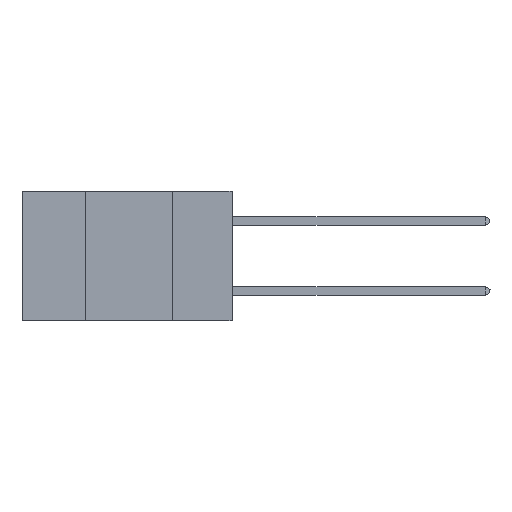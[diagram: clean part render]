
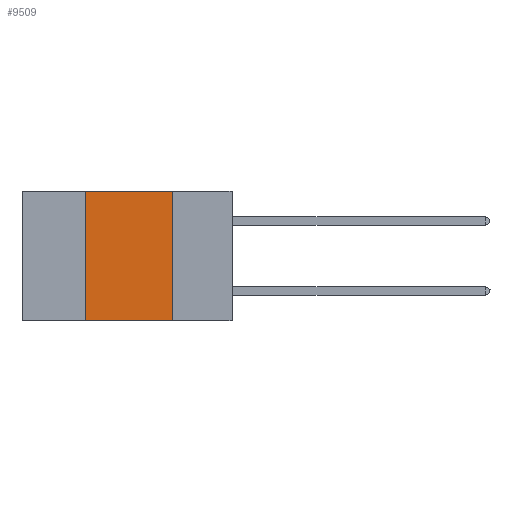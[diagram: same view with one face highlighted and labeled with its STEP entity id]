
A CAD part, left-side view. The second image highlights one B-rep face of the part: STEP entity #9509.
In plain terms, the highlighted planar face has unit normal (-1, 0, 0).
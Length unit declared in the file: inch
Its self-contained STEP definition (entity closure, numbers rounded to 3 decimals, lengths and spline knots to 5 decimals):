
#65 = DIRECTION ( 'NONE',  ( 0., -1., 0. ) ) ;
#109 = DIRECTION ( 'NONE',  ( 0., 0., -1. ) ) ;
#229 = VERTEX_POINT ( 'NONE', #6644 ) ;
#1941 = CARTESIAN_POINT ( 'NONE',  ( 0., 0.42, 0. ) ) ;
#2054 = VERTEX_POINT ( 'NONE', #14027 ) ;
#2383 = DIRECTION ( 'NONE',  ( 0., 0., 1. ) ) ;
#2789 = CARTESIAN_POINT ( 'NONE',  ( 0., 0.6, -0.37 ) ) ;
#3727 = VECTOR ( 'NONE', #12505, 39.37008 ) ;
#3840 = AXIS2_PLACEMENT_3D ( 'NONE', #13118, #4748, #14555 ) ;
#4183 = CARTESIAN_POINT ( 'NONE',  ( 0., 0.17, -0.37 ) ) ;
#4316 = LINE ( 'NONE', #12627, #7850 ) ;
#4524 = LINE ( 'NONE', #2789, #14394 ) ;
#4748 = DIRECTION ( 'NONE',  ( 1., 0., 0. ) ) ;
#4802 = ORIENTED_EDGE ( 'NONE', *, *, #10144, .T. ) ;
#6644 = CARTESIAN_POINT ( 'NONE',  ( 0., 0.42, -0.37 ) ) ;
#7850 = VECTOR ( 'NONE', #109, 39.37008 ) ;
#8315 = FACE_OUTER_BOUND ( 'NONE', #8778, .T. ) ;
#8761 = VERTEX_POINT ( 'NONE', #9739 ) ;
#8778 = EDGE_LOOP ( 'NONE', ( #17605, #14218, #14602, #4802 ) ) ;
#9509 = ADVANCED_FACE ( 'NONE', ( #8315 ), #10340, .F. ) ;
#9739 = CARTESIAN_POINT ( 'NONE',  ( 0., 0.42, 0. ) ) ;
#10140 = EDGE_CURVE ( 'NONE', #2054, #14435, #4316, .T. ) ;
#10144 = EDGE_CURVE ( 'NONE', #229, #14435, #4524, .T. ) ;
#10340 = PLANE ( 'NONE',  #3840 ) ;
#10991 = CARTESIAN_POINT ( 'NONE',  ( 0., 0.6, 0. ) ) ;
#12238 = LINE ( 'NONE', #1941, #13791 ) ;
#12505 = DIRECTION ( 'NONE',  ( 0., -1., 0. ) ) ;
#12627 = CARTESIAN_POINT ( 'NONE',  ( 0., 0.17, 0. ) ) ;
#13118 = CARTESIAN_POINT ( 'NONE',  ( 0., 0.6, 0. ) ) ;
#13791 = VECTOR ( 'NONE', #2383, 39.37008 ) ;
#14027 = CARTESIAN_POINT ( 'NONE',  ( 0., 0.17, 0. ) ) ;
#14218 = ORIENTED_EDGE ( 'NONE', *, *, #15514, .F. ) ;
#14394 = VECTOR ( 'NONE', #65, 39.37008 ) ;
#14435 = VERTEX_POINT ( 'NONE', #4183 ) ;
#14555 = DIRECTION ( 'NONE',  ( 0., 0., -1. ) ) ;
#14602 = ORIENTED_EDGE ( 'NONE', *, *, #16241, .F. ) ;
#15107 = LINE ( 'NONE', #10991, #3727 ) ;
#15514 = EDGE_CURVE ( 'NONE', #8761, #2054, #15107, .T. ) ;
#16241 = EDGE_CURVE ( 'NONE', #229, #8761, #12238, .T. ) ;
#17605 = ORIENTED_EDGE ( 'NONE', *, *, #10140, .F. ) ;
